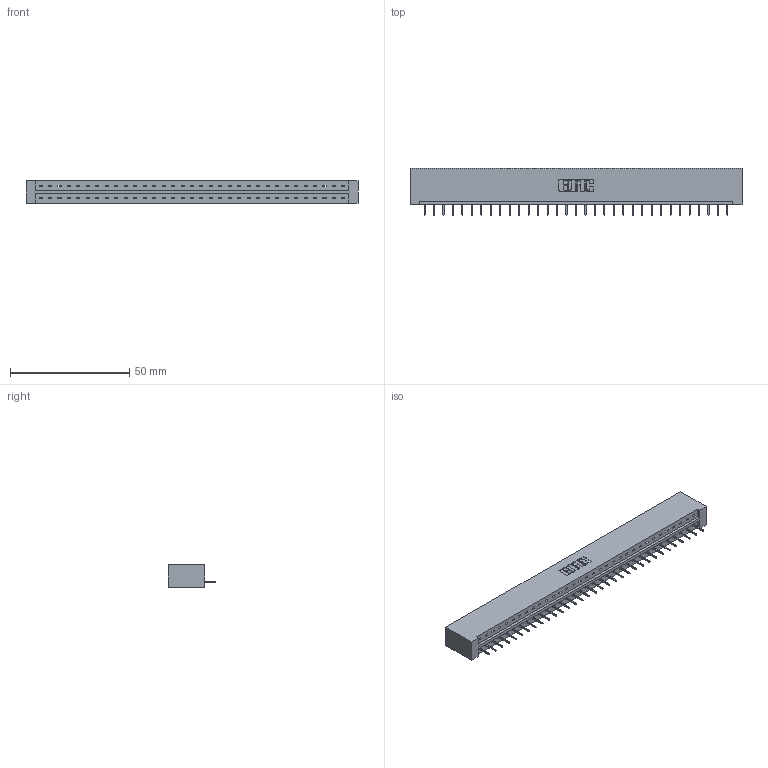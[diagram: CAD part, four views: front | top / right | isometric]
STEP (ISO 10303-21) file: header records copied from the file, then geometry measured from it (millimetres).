
FILE_DESCRIPTION (( 'STEP AP203' ), '1' );
FILE_NAME ('333-033-524-101.STEP', '2018-08-02T21:09:07', ( '' ), ( '' ), 'SwSTEP 2.0', 'SolidWorks 2016', '' );
FILE_SCHEMA (( 'CONFIG_CONTROL_DESIGN' ));
Length unit declared in the file: inch
Products named in the file (3): 333 Part_Lugless; 345-292-001_345-293-124; 333-033-524-101
Assembly tree (34 placements, depth 2):
  333-033-524-101
    333 Part_Lugless
    345-292-001_345-293-124  x33
Bounding box: 139.01 x 19.69 x 9.4 mm (x, y, z)
Volume: 14393.7 mm3; surface area: 15023.4 mm2
Topology: 34 solids, 34 shells, 2152 faces, 6227 edges, 4018 vertices
Faces by surface type: plane 1650, cylinder 502
Entity records: 21135 total; most frequent: CARTESIAN_POINT 3653, ORIENTED_EDGE 3622, DIRECTION 3093, EDGE_CURVE 1811, LINE 1695, VECTOR 1695, VERTEX_POINT 1202, AXIS2_PLACEMENT_3D 699
